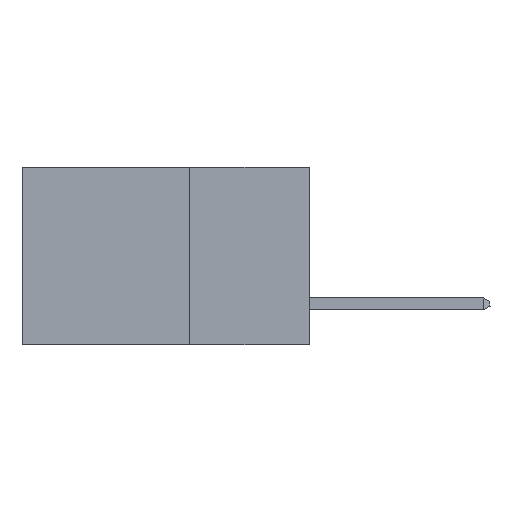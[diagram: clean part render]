
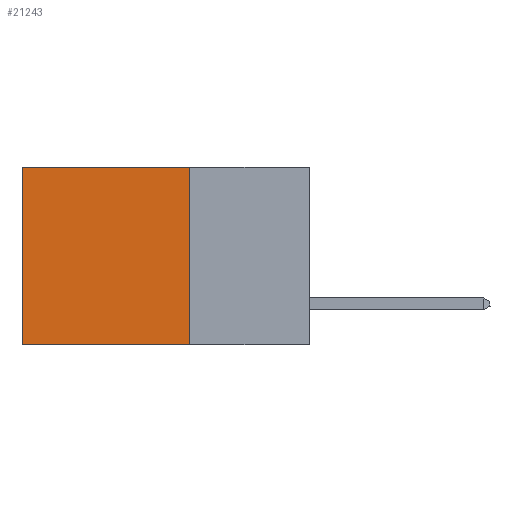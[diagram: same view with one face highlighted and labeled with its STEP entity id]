
A CAD part, left-side view. The second image highlights one B-rep face of the part: STEP entity #21243.
In plain terms, the highlighted planar face has unit normal (-1, 0, 0).
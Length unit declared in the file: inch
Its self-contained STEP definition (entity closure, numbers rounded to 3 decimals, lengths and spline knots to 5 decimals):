
#1195 = DIRECTION ( 'NONE',  ( 0., 1., 0. ) ) ;
#1559 = LINE ( 'NONE', #28518, #19840 ) ;
#2388 = EDGE_CURVE ( 'NONE', #26462, #23801, #30925, .T. ) ;
#4565 = DIRECTION ( 'NONE',  ( 1., 0., 0. ) ) ;
#4589 = EDGE_CURVE ( 'NONE', #26462, #9522, #1559, .T. ) ;
#4790 = VECTOR ( 'NONE', #22730, 39.37008 ) ;
#5090 = CARTESIAN_POINT ( 'NONE',  ( 0.2875, 0.25, 0. ) ) ;
#9522 = VERTEX_POINT ( 'NONE', #14295 ) ;
#9710 = CARTESIAN_POINT ( 'NONE',  ( 0.2875, 0.6, -0.37 ) ) ;
#10863 = LINE ( 'NONE', #28398, #25312 ) ;
#11401 = VECTOR ( 'NONE', #26179, 39.37008 ) ;
#14126 = LINE ( 'NONE', #26062, #11401 ) ;
#14295 = CARTESIAN_POINT ( 'NONE',  ( 0.2875, 0.25, -0.37 ) ) ;
#14321 = CARTESIAN_POINT ( 'NONE',  ( 0.2875, 0.25, 0. ) ) ;
#16091 = DIRECTION ( 'NONE',  ( 0., 0., -1. ) ) ;
#16842 = EDGE_LOOP ( 'NONE', ( #18078, #20112, #27268, #22947 ) ) ;
#18078 = ORIENTED_EDGE ( 'NONE', *, *, #25156, .T. ) ;
#19840 = VECTOR ( 'NONE', #16091, 39.37008 ) ;
#20112 = ORIENTED_EDGE ( 'NONE', *, *, #26244, .F. ) ;
#21243 = ADVANCED_FACE ( 'NONE', ( #22135 ), #24309, .F. ) ;
#22135 = FACE_OUTER_BOUND ( 'NONE', #16842, .T. ) ;
#22730 = DIRECTION ( 'NONE',  ( 0., 1., 0. ) ) ;
#22947 = ORIENTED_EDGE ( 'NONE', *, *, #2388, .T. ) ;
#23801 = VERTEX_POINT ( 'NONE', #29424 ) ;
#24309 = PLANE ( 'NONE',  #26486 ) ;
#25156 = EDGE_CURVE ( 'NONE', #23801, #26537, #14126, .T. ) ;
#25312 = VECTOR ( 'NONE', #1195, 39.37008 ) ;
#26062 = CARTESIAN_POINT ( 'NONE',  ( 0.2875, 0.6, 0. ) ) ;
#26179 = DIRECTION ( 'NONE',  ( 0., 0., -1. ) ) ;
#26244 = EDGE_CURVE ( 'NONE', #9522, #26537, #10863, .T. ) ;
#26462 = VERTEX_POINT ( 'NONE', #14321 ) ;
#26486 = AXIS2_PLACEMENT_3D ( 'NONE', #27052, #4565, #29860 ) ;
#26537 = VERTEX_POINT ( 'NONE', #9710 ) ;
#27052 = CARTESIAN_POINT ( 'NONE',  ( 0.2875, 0.25, 0. ) ) ;
#27268 = ORIENTED_EDGE ( 'NONE', *, *, #4589, .F. ) ;
#28398 = CARTESIAN_POINT ( 'NONE',  ( 0.2875, 0.25, -0.37 ) ) ;
#28518 = CARTESIAN_POINT ( 'NONE',  ( 0.2875, 0.25, 0. ) ) ;
#29424 = CARTESIAN_POINT ( 'NONE',  ( 0.2875, 0.6, 0. ) ) ;
#29860 = DIRECTION ( 'NONE',  ( 0., 0., -1. ) ) ;
#30925 = LINE ( 'NONE', #5090, #4790 ) ;
